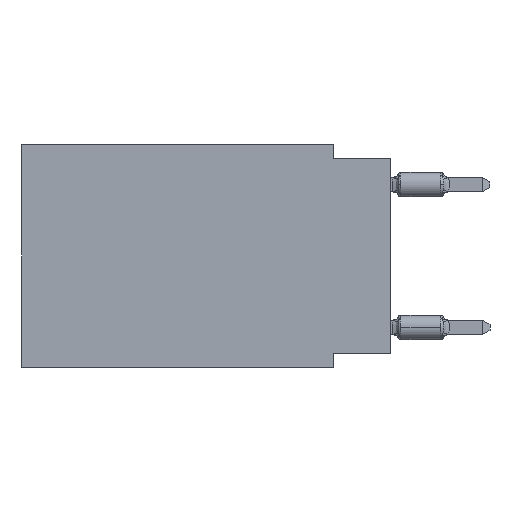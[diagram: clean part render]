
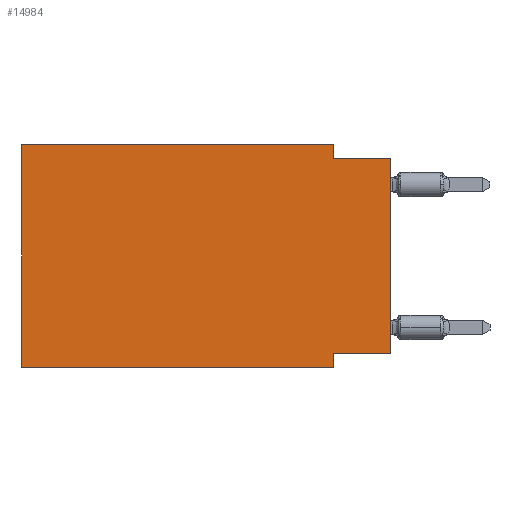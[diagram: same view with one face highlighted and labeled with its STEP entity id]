
A CAD part, left-side view. The second image highlights one B-rep face of the part: STEP entity #14984.
In plain terms, the highlighted planar face has unit normal (-1, 0, 0).
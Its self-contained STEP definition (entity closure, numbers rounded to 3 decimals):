
#132 = LINE ( 'NONE', #9515, #17147 ) ;
#159 = ORIENTED_EDGE ( 'NONE', *, *, #18072, .F. ) ;
#269 = DIRECTION ( 'NONE',  ( 0., 0., -1. ) ) ;
#495 = CARTESIAN_POINT ( 'NONE',  ( 0., 2.54, -9.906 ) ) ;
#557 = LINE ( 'NONE', #23123, #19454 ) ;
#605 = VERTEX_POINT ( 'NONE', #16039 ) ;
#909 = DIRECTION ( 'NONE',  ( 0., 0., 1. ) ) ;
#981 = LINE ( 'NONE', #24134, #8419 ) ;
#1978 = ORIENTED_EDGE ( 'NONE', *, *, #18929, .F. ) ;
#2995 = VECTOR ( 'NONE', #10446, 1000. ) ;
#3099 = EDGE_CURVE ( 'NONE', #9861, #23724, #17754, .T. ) ;
#4432 = VERTEX_POINT ( 'NONE', #19724 ) ;
#4530 = ORIENTED_EDGE ( 'NONE', *, *, #16177, .T. ) ;
#4542 = LINE ( 'NONE', #19600, #9560 ) ;
#5149 = DIRECTION ( 'NONE',  ( 0., -1., 0. ) ) ;
#5969 = DIRECTION ( 'NONE',  ( 0., -1., 0. ) ) ;
#6408 = DIRECTION ( 'NONE',  ( 0., 1., 0. ) ) ;
#6658 = CARTESIAN_POINT ( 'NONE',  ( 0., 0., -9.271 ) ) ;
#6842 = CARTESIAN_POINT ( 'NONE',  ( 0., 2.54, 0. ) ) ;
#7050 = ORIENTED_EDGE ( 'NONE', *, *, #18170, .F. ) ;
#7385 = CARTESIAN_POINT ( 'NONE',  ( 0., 2.54, -9.906 ) ) ;
#8419 = VECTOR ( 'NONE', #9236, 1000. ) ;
#9111 = CARTESIAN_POINT ( 'NONE',  ( 0., 0., -9.271 ) ) ;
#9236 = DIRECTION ( 'NONE',  ( 0., -1., 0. ) ) ;
#9419 = VECTOR ( 'NONE', #6408, 1000. ) ;
#9515 = CARTESIAN_POINT ( 'NONE',  ( 0., 2.54, 0. ) ) ;
#9560 = VECTOR ( 'NONE', #5149, 1000. ) ;
#9638 = VECTOR ( 'NONE', #5969, 1000. ) ;
#9861 = VERTEX_POINT ( 'NONE', #9111 ) ;
#10446 = DIRECTION ( 'NONE',  ( 0., 0., 1. ) ) ;
#10840 = VERTEX_POINT ( 'NONE', #22932 ) ;
#10856 = VERTEX_POINT ( 'NONE', #495 ) ;
#11735 = AXIS2_PLACEMENT_3D ( 'NONE', #21268, #11905, #19429 ) ;
#11905 = DIRECTION ( 'NONE',  ( 1., 0., 0. ) ) ;
#12164 = EDGE_LOOP ( 'NONE', ( #4530, #17514, #159, #22860, #1978, #20426, #7050, #18969 ) ) ;
#12273 = FACE_OUTER_BOUND ( 'NONE', #12164, .T. ) ;
#13015 = CARTESIAN_POINT ( 'NONE',  ( 0., 2.54, -0.635 ) ) ;
#14276 = CARTESIAN_POINT ( 'NONE',  ( 0., 16.383, 0. ) ) ;
#14984 = ADVANCED_FACE ( 'NONE', ( #12273 ), #23118, .F. ) ;
#16039 = CARTESIAN_POINT ( 'NONE',  ( 0., 16.383, 0. ) ) ;
#16128 = LINE ( 'NONE', #14276, #2995 ) ;
#16177 = EDGE_CURVE ( 'NONE', #9861, #4432, #557, .T. ) ;
#16346 = VERTEX_POINT ( 'NONE', #6842 ) ;
#17147 = VECTOR ( 'NONE', #269, 1000. ) ;
#17161 = EDGE_CURVE ( 'NONE', #20695, #4432, #981, .T. ) ;
#17514 = ORIENTED_EDGE ( 'NONE', *, *, #17161, .F. ) ;
#17649 = EDGE_CURVE ( 'NONE', #10840, #10856, #20767, .T. ) ;
#17754 = LINE ( 'NONE', #6658, #9419 ) ;
#18072 = EDGE_CURVE ( 'NONE', #16346, #20695, #132, .T. ) ;
#18170 = EDGE_CURVE ( 'NONE', #23724, #10856, #20197, .T. ) ;
#18681 = CARTESIAN_POINT ( 'NONE',  ( 0., 16.383, -9.906 ) ) ;
#18929 = EDGE_CURVE ( 'NONE', #10840, #605, #16128, .T. ) ;
#18969 = ORIENTED_EDGE ( 'NONE', *, *, #3099, .F. ) ;
#19429 = DIRECTION ( 'NONE',  ( 0., 0., -1. ) ) ;
#19454 = VECTOR ( 'NONE', #909, 1000. ) ;
#19600 = CARTESIAN_POINT ( 'NONE',  ( 0., 16.383, 0. ) ) ;
#19724 = CARTESIAN_POINT ( 'NONE',  ( 0., 0., -0.635 ) ) ;
#20197 = LINE ( 'NONE', #7385, #21074 ) ;
#20227 = EDGE_CURVE ( 'NONE', #605, #16346, #4542, .T. ) ;
#20426 = ORIENTED_EDGE ( 'NONE', *, *, #17649, .T. ) ;
#20695 = VERTEX_POINT ( 'NONE', #13015 ) ;
#20767 = LINE ( 'NONE', #18681, #9638 ) ;
#21074 = VECTOR ( 'NONE', #24249, 1000. ) ;
#21268 = CARTESIAN_POINT ( 'NONE',  ( 0., 16.383, 0. ) ) ;
#22860 = ORIENTED_EDGE ( 'NONE', *, *, #20227, .F. ) ;
#22932 = CARTESIAN_POINT ( 'NONE',  ( 0., 16.383, -9.906 ) ) ;
#23118 = PLANE ( 'NONE',  #11735 ) ;
#23123 = CARTESIAN_POINT ( 'NONE',  ( 0., 0., 0. ) ) ;
#23689 = CARTESIAN_POINT ( 'NONE',  ( 0., 2.54, -9.271 ) ) ;
#23724 = VERTEX_POINT ( 'NONE', #23689 ) ;
#24134 = CARTESIAN_POINT ( 'NONE',  ( 0., 0., -0.635 ) ) ;
#24249 = DIRECTION ( 'NONE',  ( 0., 0., -1. ) ) ;
